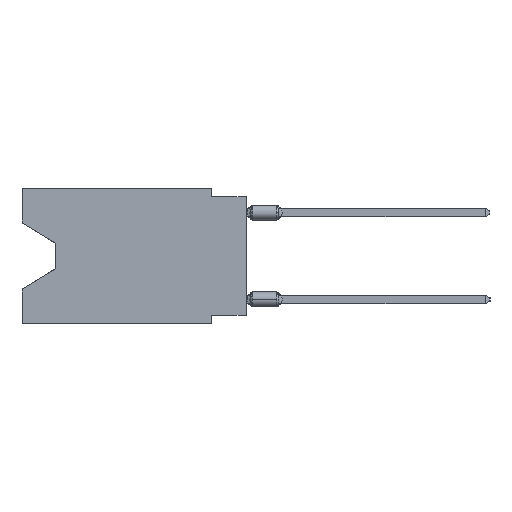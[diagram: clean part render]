
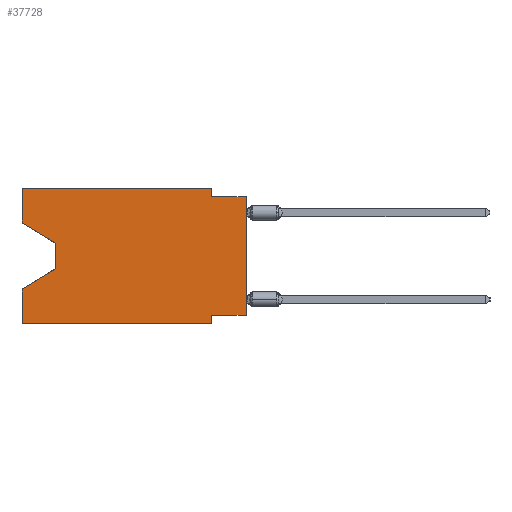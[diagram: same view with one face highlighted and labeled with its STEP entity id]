
A CAD part, left-side view. The second image highlights one B-rep face of the part: STEP entity #37728.
In plain terms, the highlighted planar face has unit normal (-1, 0, 0).
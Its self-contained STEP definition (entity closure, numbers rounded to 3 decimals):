
#233 = DIRECTION ( 'NONE',  ( 0., 0., 1. ) ) ;
#308 = LINE ( 'NONE', #4267, #20153 ) ;
#719 = DIRECTION ( 'NONE',  ( 0., -1., 0. ) ) ;
#870 = DIRECTION ( 'NONE',  ( 0., 0., -1. ) ) ;
#1564 = LINE ( 'NONE', #29056, #42846 ) ;
#1598 = DIRECTION ( 'NONE',  ( 0., 0., -1. ) ) ;
#4053 = VERTEX_POINT ( 'NONE', #46108 ) ;
#4267 = CARTESIAN_POINT ( 'NONE',  ( 0., 16.383, 0. ) ) ;
#4764 = VERTEX_POINT ( 'NONE', #25066 ) ;
#5004 = CARTESIAN_POINT ( 'NONE',  ( 0., 2.54, -0.635 ) ) ;
#5350 = LINE ( 'NONE', #29911, #49167 ) ;
#6619 = VERTEX_POINT ( 'NONE', #11402 ) ;
#7017 = EDGE_CURVE ( 'NONE', #39816, #45524, #41743, .T. ) ;
#7673 = DIRECTION ( 'NONE',  ( 0., 0., -1. ) ) ;
#8521 = AXIS2_PLACEMENT_3D ( 'NONE', #29394, #44993, #870 ) ;
#10220 = VERTEX_POINT ( 'NONE', #48519 ) ;
#11104 = DIRECTION ( 'NONE',  ( 0., 1., 0. ) ) ;
#11269 = ORIENTED_EDGE ( 'NONE', *, *, #32376, .F. ) ;
#11402 = CARTESIAN_POINT ( 'NONE',  ( 0., 0., -9.271 ) ) ;
#11423 = VERTEX_POINT ( 'NONE', #48780 ) ;
#12590 = LINE ( 'NONE', #20780, #18102 ) ;
#12810 = EDGE_CURVE ( 'NONE', #4053, #10220, #45680, .T. ) ;
#14258 = ORIENTED_EDGE ( 'NONE', *, *, #12810, .F. ) ;
#14695 = VERTEX_POINT ( 'NONE', #45843 ) ;
#15311 = LINE ( 'NONE', #39082, #25260 ) ;
#15546 = ORIENTED_EDGE ( 'NONE', *, *, #49498, .F. ) ;
#15585 = VERTEX_POINT ( 'NONE', #23250 ) ;
#16719 = VECTOR ( 'NONE', #233, 1000. ) ;
#17244 = PLANE ( 'NONE',  #8521 ) ;
#17656 = ORIENTED_EDGE ( 'NONE', *, *, #19955, .T. ) ;
#18102 = VECTOR ( 'NONE', #719, 1000. ) ;
#19955 = EDGE_CURVE ( 'NONE', #4764, #11423, #28015, .T. ) ;
#20007 = LINE ( 'NONE', #36122, #50036 ) ;
#20147 = VECTOR ( 'NONE', #34296, 1000. ) ;
#20153 = VECTOR ( 'NONE', #48385, 1000. ) ;
#20551 = LINE ( 'NONE', #27715, #16719 ) ;
#20780 = CARTESIAN_POINT ( 'NONE',  ( 0., 16.383, 0. ) ) ;
#21858 = VECTOR ( 'NONE', #11104, 1000. ) ;
#22627 = CARTESIAN_POINT ( 'NONE',  ( 0., 2.54, 0. ) ) ;
#22697 = DIRECTION ( 'NONE',  ( 0., 0.855, -0.519 ) ) ;
#23040 = EDGE_CURVE ( 'NONE', #4053, #15585, #35204, .T. ) ;
#23250 = CARTESIAN_POINT ( 'NONE',  ( 0., 2.54, -9.906 ) ) ;
#25066 = CARTESIAN_POINT ( 'NONE',  ( 0., 13.97, -4.013 ) ) ;
#25260 = VECTOR ( 'NONE', #22697, 1000. ) ;
#27715 = CARTESIAN_POINT ( 'NONE',  ( 0., 0., 0. ) ) ;
#28015 = LINE ( 'NONE', #31713, #45110 ) ;
#28185 = VERTEX_POINT ( 'NONE', #51669 ) ;
#28790 = DIRECTION ( 'NONE',  ( 0., -1., 0. ) ) ;
#28884 = FACE_OUTER_BOUND ( 'NONE', #32770, .T. ) ;
#29056 = CARTESIAN_POINT ( 'NONE',  ( 0., 0., -0.635 ) ) ;
#29394 = CARTESIAN_POINT ( 'NONE',  ( 0., 16.383, 0. ) ) ;
#29661 = DIRECTION ( 'NONE',  ( 0., 0., -1. ) ) ;
#29911 = CARTESIAN_POINT ( 'NONE',  ( 0., 2.54, -9.906 ) ) ;
#30588 = EDGE_CURVE ( 'NONE', #6619, #28185, #38566, .T. ) ;
#30718 = VECTOR ( 'NONE', #1598, 1000. ) ;
#31190 = ORIENTED_EDGE ( 'NONE', *, *, #30588, .F. ) ;
#31713 = CARTESIAN_POINT ( 'NONE',  ( 0., 13.97, -4.013 ) ) ;
#32376 = EDGE_CURVE ( 'NONE', #14695, #39816, #12590, .T. ) ;
#32770 = EDGE_LOOP ( 'NONE', ( #42704, #17656, #38672, #14258, #50043, #40267, #31190, #46072, #15546, #34084, #11269, #35665 ) ) ;
#33783 = CARTESIAN_POINT ( 'NONE',  ( 0., 16.383, 0. ) ) ;
#34084 = ORIENTED_EDGE ( 'NONE', *, *, #7017, .F. ) ;
#34296 = DIRECTION ( 'NONE',  ( 0., 0., 1. ) ) ;
#34415 = EDGE_CURVE ( 'NONE', #6619, #50492, #20551, .T. ) ;
#35204 = LINE ( 'NONE', #43146, #40165 ) ;
#35280 = EDGE_CURVE ( 'NONE', #38650, #14695, #308, .T. ) ;
#35475 = DIRECTION ( 'NONE',  ( 0., -1., 0. ) ) ;
#35578 = EDGE_CURVE ( 'NONE', #11423, #10220, #15311, .T. ) ;
#35665 = ORIENTED_EDGE ( 'NONE', *, *, #35280, .F. ) ;
#35666 = CARTESIAN_POINT ( 'NONE',  ( 0., 0., -9.271 ) ) ;
#36122 = CARTESIAN_POINT ( 'NONE',  ( 0., 16.383, -2.546 ) ) ;
#37728 = ADVANCED_FACE ( 'NONE', ( #28884 ), #17244, .F. ) ;
#38566 = LINE ( 'NONE', #35666, #21858 ) ;
#38650 = VERTEX_POINT ( 'NONE', #46864 ) ;
#38672 = ORIENTED_EDGE ( 'NONE', *, *, #35578, .T. ) ;
#39082 = CARTESIAN_POINT ( 'NONE',  ( 0., 13.97, -5.893 ) ) ;
#39816 = VERTEX_POINT ( 'NONE', #22627 ) ;
#40165 = VECTOR ( 'NONE', #35475, 1000. ) ;
#40267 = ORIENTED_EDGE ( 'NONE', *, *, #44708, .F. ) ;
#41743 = LINE ( 'NONE', #45970, #30718 ) ;
#42704 = ORIENTED_EDGE ( 'NONE', *, *, #45993, .T. ) ;
#42846 = VECTOR ( 'NONE', #28790, 1000. ) ;
#43146 = CARTESIAN_POINT ( 'NONE',  ( 0., 16.383, -9.906 ) ) ;
#44708 = EDGE_CURVE ( 'NONE', #28185, #15585, #5350, .T. ) ;
#44993 = DIRECTION ( 'NONE',  ( 1., 0., 0. ) ) ;
#45110 = VECTOR ( 'NONE', #7673, 1000. ) ;
#45524 = VERTEX_POINT ( 'NONE', #5004 ) ;
#45680 = LINE ( 'NONE', #33783, #20147 ) ;
#45843 = CARTESIAN_POINT ( 'NONE',  ( 0., 16.383, 0. ) ) ;
#45970 = CARTESIAN_POINT ( 'NONE',  ( 0., 2.54, 0. ) ) ;
#45993 = EDGE_CURVE ( 'NONE', #38650, #4764, #20007, .T. ) ;
#46072 = ORIENTED_EDGE ( 'NONE', *, *, #34415, .T. ) ;
#46108 = CARTESIAN_POINT ( 'NONE',  ( 0., 16.383, -9.906 ) ) ;
#46864 = CARTESIAN_POINT ( 'NONE',  ( 0., 16.383, -2.546 ) ) ;
#48385 = DIRECTION ( 'NONE',  ( 0., 0., 1. ) ) ;
#48519 = CARTESIAN_POINT ( 'NONE',  ( 0., 16.383, -7.36 ) ) ;
#48780 = CARTESIAN_POINT ( 'NONE',  ( 0., 13.97, -5.893 ) ) ;
#49167 = VECTOR ( 'NONE', #29661, 1000. ) ;
#49498 = EDGE_CURVE ( 'NONE', #45524, #50492, #1564, .T. ) ;
#49783 = DIRECTION ( 'NONE',  ( 0., -0.855, -0.519 ) ) ;
#50036 = VECTOR ( 'NONE', #49783, 1000. ) ;
#50043 = ORIENTED_EDGE ( 'NONE', *, *, #23040, .T. ) ;
#50492 = VERTEX_POINT ( 'NONE', #50547 ) ;
#50547 = CARTESIAN_POINT ( 'NONE',  ( 0., 0., -0.635 ) ) ;
#51669 = CARTESIAN_POINT ( 'NONE',  ( 0., 2.54, -9.271 ) ) ;
